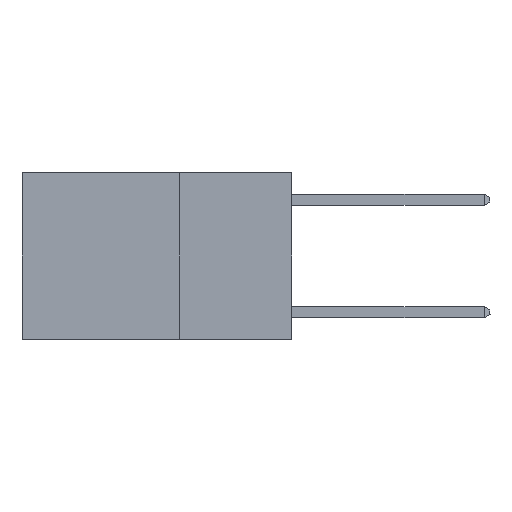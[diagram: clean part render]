
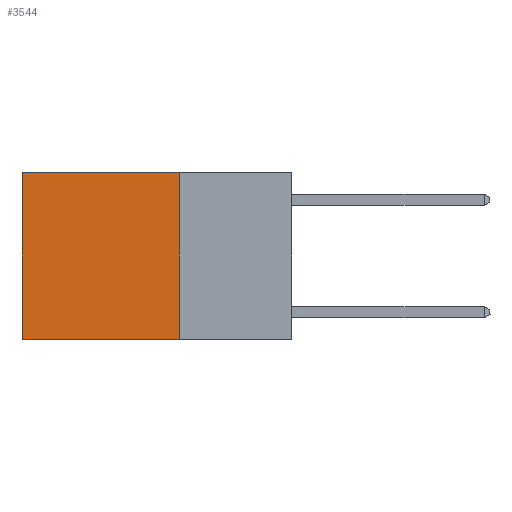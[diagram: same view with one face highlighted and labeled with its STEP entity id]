
A CAD part, left-side view. The second image highlights one B-rep face of the part: STEP entity #3544.
In plain terms, the highlighted planar face has unit normal (-1, 0, 0).
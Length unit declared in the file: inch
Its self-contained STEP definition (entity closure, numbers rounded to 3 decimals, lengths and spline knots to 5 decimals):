
#443 = LINE ( 'NONE', #2413, #2913 ) ;
#701 = DIRECTION ( 'NONE',  ( 1., 0., 0. ) ) ;
#1178 = CARTESIAN_POINT ( 'NONE',  ( 0.2625, 0.25, 0. ) ) ;
#1420 = ORIENTED_EDGE ( 'NONE', *, *, #8953, .T. ) ;
#2413 = CARTESIAN_POINT ( 'NONE',  ( 0.2625, 0.6, 0. ) ) ;
#2707 = LINE ( 'NONE', #3014, #8485 ) ;
#2828 = CARTESIAN_POINT ( 'NONE',  ( 0.2625, 0.25, -0.37 ) ) ;
#2913 = VECTOR ( 'NONE', #11904, 39.37008 ) ;
#3014 = CARTESIAN_POINT ( 'NONE',  ( 0.2625, 0.25, 0. ) ) ;
#3544 = ADVANCED_FACE ( 'NONE', ( #8748 ), #12252, .F. ) ;
#4341 = VERTEX_POINT ( 'NONE', #6531 ) ;
#5145 = DIRECTION ( 'NONE',  ( 0., 0., -1. ) ) ;
#5521 = CARTESIAN_POINT ( 'NONE',  ( 0.2625, 0.25, -0.37 ) ) ;
#6268 = EDGE_CURVE ( 'NONE', #4341, #7812, #2707, .T. ) ;
#6531 = CARTESIAN_POINT ( 'NONE',  ( 0.2625, 0.25, 0. ) ) ;
#7027 = ORIENTED_EDGE ( 'NONE', *, *, #10515, .T. ) ;
#7812 = VERTEX_POINT ( 'NONE', #5521 ) ;
#8091 = DIRECTION ( 'NONE',  ( 0., 0., -1. ) ) ;
#8319 = CARTESIAN_POINT ( 'NONE',  ( 0.2625, 0.6, 0. ) ) ;
#8336 = EDGE_LOOP ( 'NONE', ( #7027, #11341, #12033, #1420 ) ) ;
#8485 = VECTOR ( 'NONE', #5145, 39.37008 ) ;
#8748 = FACE_OUTER_BOUND ( 'NONE', #8336, .T. ) ;
#8953 = EDGE_CURVE ( 'NONE', #4341, #10233, #12031, .T. ) ;
#9590 = VECTOR ( 'NONE', #9652, 39.37008 ) ;
#9652 = DIRECTION ( 'NONE',  ( 0., 1., 0. ) ) ;
#10100 = EDGE_CURVE ( 'NONE', #7812, #11974, #13429, .T. ) ;
#10233 = VERTEX_POINT ( 'NONE', #8319 ) ;
#10380 = VECTOR ( 'NONE', #13287, 39.37008 ) ;
#10515 = EDGE_CURVE ( 'NONE', #10233, #11974, #443, .T. ) ;
#11119 = CARTESIAN_POINT ( 'NONE',  ( 0.2625, 0.6, -0.37 ) ) ;
#11341 = ORIENTED_EDGE ( 'NONE', *, *, #10100, .F. ) ;
#11904 = DIRECTION ( 'NONE',  ( 0., 0., -1. ) ) ;
#11974 = VERTEX_POINT ( 'NONE', #11119 ) ;
#12031 = LINE ( 'NONE', #1178, #9590 ) ;
#12033 = ORIENTED_EDGE ( 'NONE', *, *, #6268, .F. ) ;
#12252 = PLANE ( 'NONE',  #12344 ) ;
#12344 = AXIS2_PLACEMENT_3D ( 'NONE', #13276, #701, #8091 ) ;
#13276 = CARTESIAN_POINT ( 'NONE',  ( 0.2625, 0.25, 0. ) ) ;
#13287 = DIRECTION ( 'NONE',  ( 0., 1., 0. ) ) ;
#13429 = LINE ( 'NONE', #2828, #10380 ) ;
